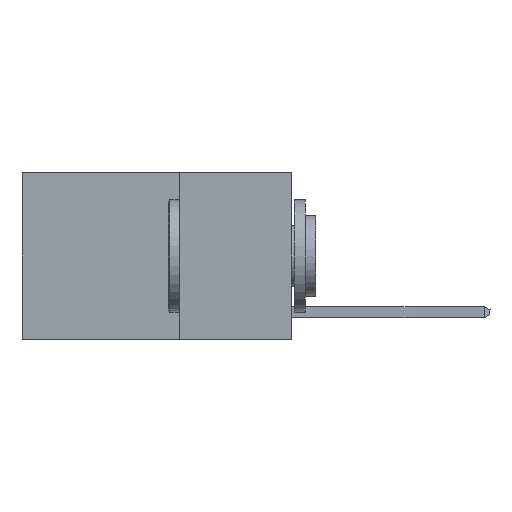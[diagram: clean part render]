
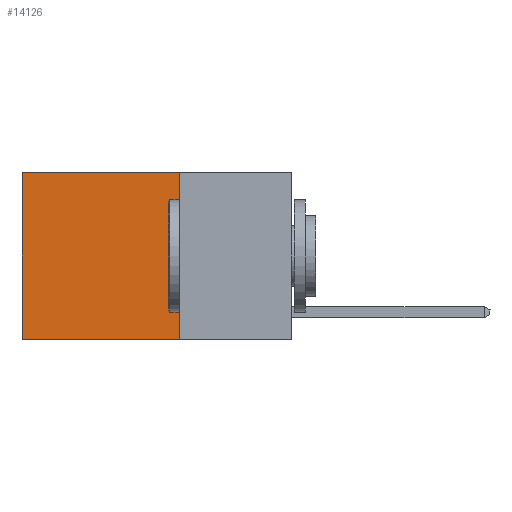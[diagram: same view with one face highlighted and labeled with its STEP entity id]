
A CAD part, left-side view. The second image highlights one B-rep face of the part: STEP entity #14126.
In plain terms, the highlighted planar face has unit normal (-1, 0, 0).
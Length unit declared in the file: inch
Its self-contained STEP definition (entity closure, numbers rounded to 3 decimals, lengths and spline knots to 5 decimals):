
#1573 = LINE ( 'NONE', #7175, #12013 ) ;
#2546 = CARTESIAN_POINT ( 'NONE',  ( 0.2625, 0.25, 0. ) ) ;
#2784 = ORIENTED_EDGE ( 'NONE', *, *, #9503, .F. ) ;
#2940 = EDGE_CURVE ( 'NONE', #9894, #15812, #5227, .T. ) ;
#3674 = EDGE_CURVE ( 'NONE', #7225, #8823, #7145, .T. ) ;
#5227 = LINE ( 'NONE', #14991, #5254 ) ;
#5254 = VECTOR ( 'NONE', #10663, 39.37008 ) ;
#5959 = CARTESIAN_POINT ( 'NONE',  ( 0.2625, 0.25, 0. ) ) ;
#6540 = DIRECTION ( 'NONE',  ( 0., 1., 0. ) ) ;
#7145 = LINE ( 'NONE', #5959, #16861 ) ;
#7175 = CARTESIAN_POINT ( 'NONE',  ( 0.2625, 0.25, -0.37 ) ) ;
#7225 = VERTEX_POINT ( 'NONE', #2546 ) ;
#7923 = CARTESIAN_POINT ( 'NONE',  ( 0.2625, 0.6, -0.37 ) ) ;
#7930 = LINE ( 'NONE', #13585, #17693 ) ;
#8403 = PLANE ( 'NONE',  #11809 ) ;
#8823 = VERTEX_POINT ( 'NONE', #11212 ) ;
#9503 = EDGE_CURVE ( 'NONE', #8823, #15812, #1573, .T. ) ;
#9894 = VERTEX_POINT ( 'NONE', #14302 ) ;
#10663 = DIRECTION ( 'NONE',  ( 0., 0., -1. ) ) ;
#11212 = CARTESIAN_POINT ( 'NONE',  ( 0.2625, 0.25, -0.37 ) ) ;
#11286 = FACE_OUTER_BOUND ( 'NONE', #17782, .T. ) ;
#11419 = EDGE_CURVE ( 'NONE', #7225, #9894, #7930, .T. ) ;
#11628 = DIRECTION ( 'NONE',  ( 0., 0., -1. ) ) ;
#11809 = AXIS2_PLACEMENT_3D ( 'NONE', #12494, #15365, #12763 ) ;
#12013 = VECTOR ( 'NONE', #16964, 39.37008 ) ;
#12494 = CARTESIAN_POINT ( 'NONE',  ( 0.2625, 0.25, 0. ) ) ;
#12763 = DIRECTION ( 'NONE',  ( 0., 0., -1. ) ) ;
#13585 = CARTESIAN_POINT ( 'NONE',  ( 0.2625, 0.25, 0. ) ) ;
#13963 = ORIENTED_EDGE ( 'NONE', *, *, #3674, .F. ) ;
#14126 = ADVANCED_FACE ( 'NONE', ( #11286 ), #8403, .F. ) ;
#14302 = CARTESIAN_POINT ( 'NONE',  ( 0.2625, 0.6, 0. ) ) ;
#14991 = CARTESIAN_POINT ( 'NONE',  ( 0.2625, 0.6, 0. ) ) ;
#15265 = ORIENTED_EDGE ( 'NONE', *, *, #2940, .T. ) ;
#15365 = DIRECTION ( 'NONE',  ( 1., 0., 0. ) ) ;
#15812 = VERTEX_POINT ( 'NONE', #7923 ) ;
#16861 = VECTOR ( 'NONE', #11628, 39.37008 ) ;
#16964 = DIRECTION ( 'NONE',  ( 0., 1., 0. ) ) ;
#17682 = ORIENTED_EDGE ( 'NONE', *, *, #11419, .T. ) ;
#17693 = VECTOR ( 'NONE', #6540, 39.37008 ) ;
#17782 = EDGE_LOOP ( 'NONE', ( #15265, #2784, #13963, #17682 ) ) ;
